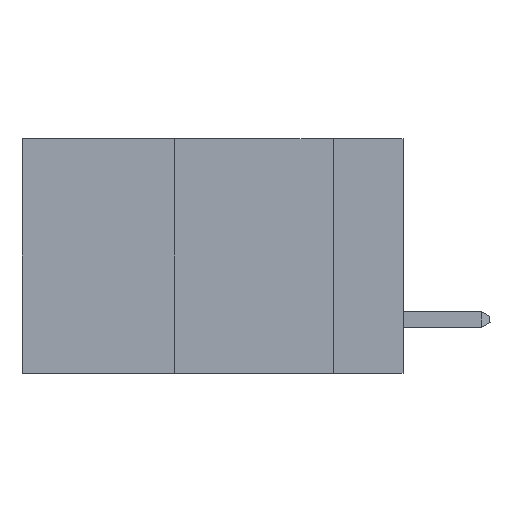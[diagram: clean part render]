
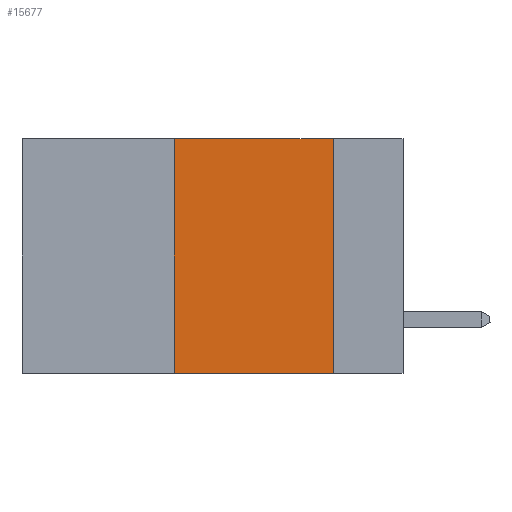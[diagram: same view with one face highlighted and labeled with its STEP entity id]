
A CAD part, left-side view. The second image highlights one B-rep face of the part: STEP entity #15677.
In plain terms, the highlighted planar face has unit normal (-1, 0, 0).
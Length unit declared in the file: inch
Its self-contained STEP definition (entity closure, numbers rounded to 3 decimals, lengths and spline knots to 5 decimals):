
#262 = EDGE_LOOP ( 'NONE', ( #14730, #1688, #1322, #6441 ) ) ;
#410 = VECTOR ( 'NONE', #14215, 39.37008 ) ;
#712 = CARTESIAN_POINT ( 'NONE',  ( 0., 0.36, 0. ) ) ;
#815 = LINE ( 'NONE', #15409, #410 ) ;
#854 = VERTEX_POINT ( 'NONE', #14786 ) ;
#1307 = LINE ( 'NONE', #11914, #16219 ) ;
#1322 = ORIENTED_EDGE ( 'NONE', *, *, #7473, .F. ) ;
#1688 = ORIENTED_EDGE ( 'NONE', *, *, #11307, .F. ) ;
#2247 = CARTESIAN_POINT ( 'NONE',  ( 0., 0.11, 0. ) ) ;
#2259 = CARTESIAN_POINT ( 'NONE',  ( 0., 0.36, -0.37 ) ) ;
#4274 = EDGE_CURVE ( 'NONE', #15910, #854, #815, .T. ) ;
#4470 = DIRECTION ( 'NONE',  ( 0., -1., 0. ) ) ;
#4613 = VECTOR ( 'NONE', #7958, 39.37008 ) ;
#5896 = LINE ( 'NONE', #6172, #11395 ) ;
#6172 = CARTESIAN_POINT ( 'NONE',  ( 0., 0.36, 0. ) ) ;
#6379 = EDGE_CURVE ( 'NONE', #11581, #854, #1307, .T. ) ;
#6441 = ORIENTED_EDGE ( 'NONE', *, *, #6379, .T. ) ;
#6649 = PLANE ( 'NONE',  #14517 ) ;
#6754 = CARTESIAN_POINT ( 'NONE',  ( 0., 0.6, 0. ) ) ;
#7139 = FACE_OUTER_BOUND ( 'NONE', #262, .T. ) ;
#7473 = EDGE_CURVE ( 'NONE', #11581, #15161, #5896, .T. ) ;
#7958 = DIRECTION ( 'NONE',  ( 0., -1., 0. ) ) ;
#8039 = DIRECTION ( 'NONE',  ( 0., 0., -1. ) ) ;
#11307 = EDGE_CURVE ( 'NONE', #15161, #15910, #15973, .T. ) ;
#11395 = VECTOR ( 'NONE', #16027, 39.37008 ) ;
#11581 = VERTEX_POINT ( 'NONE', #2259 ) ;
#11914 = CARTESIAN_POINT ( 'NONE',  ( 0., 0.6, -0.37 ) ) ;
#14215 = DIRECTION ( 'NONE',  ( 0., 0., -1. ) ) ;
#14293 = CARTESIAN_POINT ( 'NONE',  ( 0., 0.6, 0. ) ) ;
#14517 = AXIS2_PLACEMENT_3D ( 'NONE', #6754, #15343, #8039 ) ;
#14730 = ORIENTED_EDGE ( 'NONE', *, *, #4274, .F. ) ;
#14786 = CARTESIAN_POINT ( 'NONE',  ( 0., 0.11, -0.37 ) ) ;
#15161 = VERTEX_POINT ( 'NONE', #712 ) ;
#15343 = DIRECTION ( 'NONE',  ( 1., 0., 0. ) ) ;
#15409 = CARTESIAN_POINT ( 'NONE',  ( 0., 0.11, 0. ) ) ;
#15677 = ADVANCED_FACE ( 'NONE', ( #7139 ), #6649, .F. ) ;
#15910 = VERTEX_POINT ( 'NONE', #2247 ) ;
#15973 = LINE ( 'NONE', #14293, #4613 ) ;
#16027 = DIRECTION ( 'NONE',  ( 0., 0., 1. ) ) ;
#16219 = VECTOR ( 'NONE', #4470, 39.37008 ) ;
